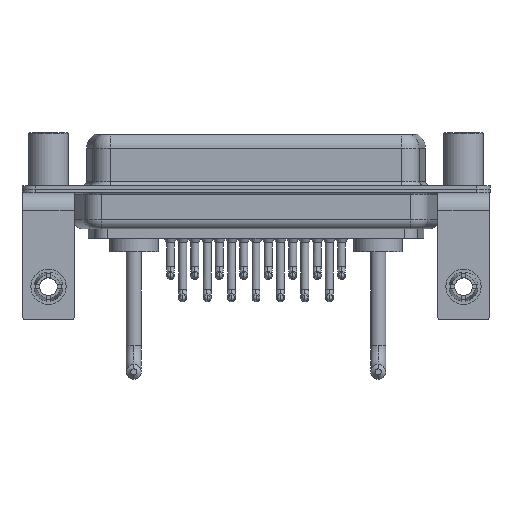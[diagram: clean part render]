
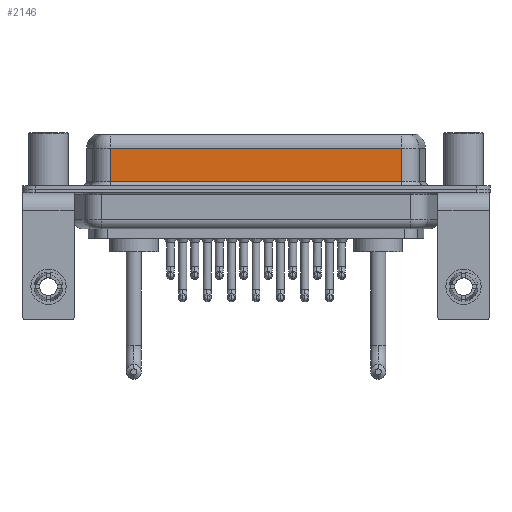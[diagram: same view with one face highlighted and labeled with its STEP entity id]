
A CAD part, front view. The second image highlights one B-rep face of the part: STEP entity #2146.
In plain terms, the highlighted planar face has unit normal (0, -1, 0).
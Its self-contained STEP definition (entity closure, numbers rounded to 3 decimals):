
#2146 = ADVANCED_FACE ( 'NONE', ( #11251 ), #13262, .F. ) ;
#2938 = CARTESIAN_POINT ( 'NONE',  ( 40.037, -3.95, 4.65 ) ) ;
#3031 = CARTESIAN_POINT ( 'NONE',  ( 40.037, -3.95, 6.4 ) ) ;
#4147 = EDGE_LOOP ( 'NONE', ( #11948, #8237, #11019, #17299 ) ) ;
#4839 = DIRECTION ( 'NONE',  ( -1., 0., 0. ) ) ;
#5427 = DIRECTION ( 'NONE',  ( 0., 0., 1. ) ) ;
#5972 = VERTEX_POINT ( 'NONE', #24742 ) ;
#6122 = EDGE_CURVE ( 'NONE', #21657, #18302, #13850, .T. ) ;
#6414 = VERTEX_POINT ( 'NONE', #11301 ) ;
#6529 = LINE ( 'NONE', #16630, #18912 ) ;
#6562 = LINE ( 'NONE', #8566, #10458 ) ;
#7851 = AXIS2_PLACEMENT_3D ( 'NONE', #3031, #14917, #5427 ) ;
#8237 = ORIENTED_EDGE ( 'NONE', *, *, #13525, .T. ) ;
#8566 = CARTESIAN_POINT ( 'NONE',  ( 40.037, -3.95, 0.9 ) ) ;
#8904 = DIRECTION ( 'NONE',  ( 0., 0., -1. ) ) ;
#10458 = VECTOR ( 'NONE', #18435, 1000. ) ;
#11019 = ORIENTED_EDGE ( 'NONE', *, *, #22177, .T. ) ;
#11251 = FACE_OUTER_BOUND ( 'NONE', #4147, .T. ) ;
#11301 = CARTESIAN_POINT ( 'NONE',  ( 7.013, -3.95, 0.9 ) ) ;
#11948 = ORIENTED_EDGE ( 'NONE', *, *, #6122, .F. ) ;
#12983 = EDGE_CURVE ( 'NONE', #6414, #18302, #6562, .T. ) ;
#13262 = PLANE ( 'NONE',  #7851 ) ;
#13525 = EDGE_CURVE ( 'NONE', #21657, #5972, #22165, .T. ) ;
#13800 = CARTESIAN_POINT ( 'NONE',  ( 40.037, -3.95, 4.65 ) ) ;
#13850 = LINE ( 'NONE', #13977, #19124 ) ;
#13977 = CARTESIAN_POINT ( 'NONE',  ( 40.037, -3.95, 6.4 ) ) ;
#14125 = CARTESIAN_POINT ( 'NONE',  ( 40.037, -3.95, 0.9 ) ) ;
#14917 = DIRECTION ( 'NONE',  ( 0., 1., 0. ) ) ;
#16630 = CARTESIAN_POINT ( 'NONE',  ( 7.013, -3.95, 6.4 ) ) ;
#17299 = ORIENTED_EDGE ( 'NONE', *, *, #12983, .T. ) ;
#18302 = VERTEX_POINT ( 'NONE', #14125 ) ;
#18435 = DIRECTION ( 'NONE',  ( 1., 0., 0. ) ) ;
#18912 = VECTOR ( 'NONE', #8904, 1000. ) ;
#19124 = VECTOR ( 'NONE', #21692, 1000. ) ;
#21657 = VERTEX_POINT ( 'NONE', #13800 ) ;
#21692 = DIRECTION ( 'NONE',  ( 0., 0., -1. ) ) ;
#22165 = LINE ( 'NONE', #2938, #23352 ) ;
#22177 = EDGE_CURVE ( 'NONE', #5972, #6414, #6529, .T. ) ;
#23352 = VECTOR ( 'NONE', #4839, 1000. ) ;
#24742 = CARTESIAN_POINT ( 'NONE',  ( 7.013, -3.95, 4.65 ) ) ;
